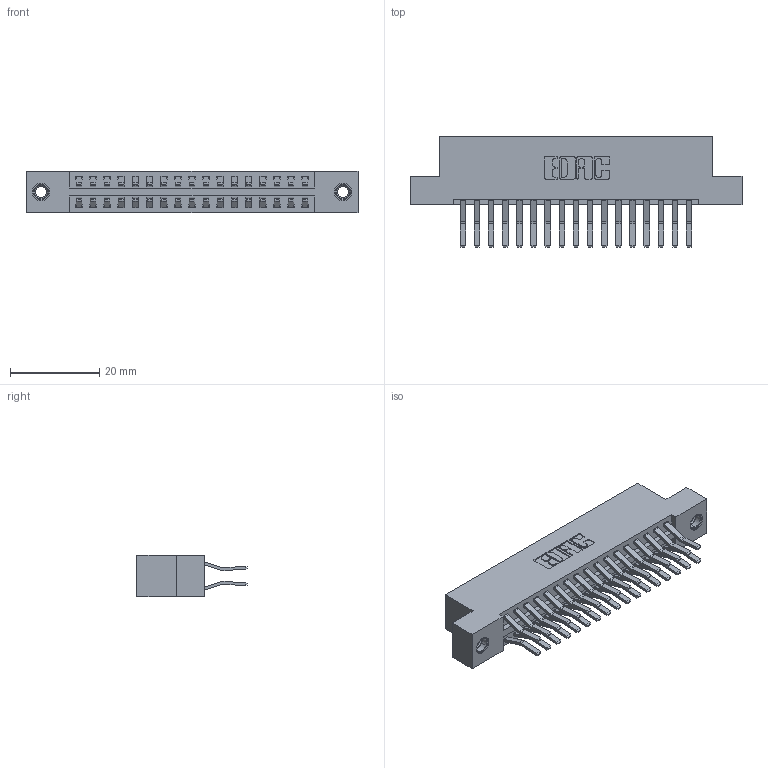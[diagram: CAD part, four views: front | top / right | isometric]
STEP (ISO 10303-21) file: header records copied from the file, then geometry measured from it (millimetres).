
FILE_DESCRIPTION (( 'STEP AP203' ), '1' );
FILE_NAME ('346-034-560-207.STEP', '2018-08-23T23:32:04', ( '' ), ( '' ), 'SwSTEP 2.0', 'SolidWorks 2016', '' );
FILE_SCHEMA (( 'CONFIG_CONTROL_DESIGN' ));
Length unit declared in the file: inch
Products named in the file (4): 345-250-001_345-250-005-103; 346-034-560-207; 346 Part_Flush Mounting Lugs - 0.156 Dia-TI; 345-292-001_560 Tail
Assembly tree (37 placements, depth 2):
  346-034-560-207
    346 Part_Flush Mounting Lugs - 0.156 Dia-TI
    345-292-001_560 Tail  x34
    345-250-001_345-250-005-103  x2
Bounding box: 74.55 x 24.78 x 9.4 mm (x, y, z)
Volume: 7284.6 mm3; surface area: 10248.6 mm2
Topology: 37 solids, 37 shells, 2018 faces, 5939 edges, 3906 vertices
Faces by surface type: plane 1298, cylinder 704, cone 12, torus 4
Entity records: 15734 total; most frequent: CARTESIAN_POINT 2611, ORIENTED_EDGE 2538, DIRECTION 2383, EDGE_CURVE 1269, LINE 1045, VECTOR 1045, VERTEX_POINT 840, AXIS2_PLACEMENT_3D 669
